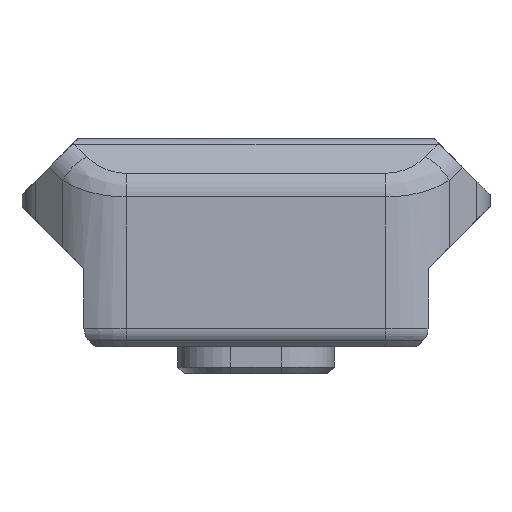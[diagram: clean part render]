
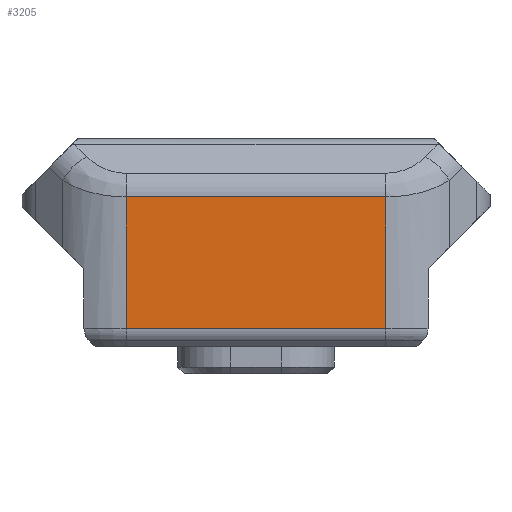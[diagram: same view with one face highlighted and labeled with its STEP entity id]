
A CAD part, front view. The second image highlights one B-rep face of the part: STEP entity #3205.
In plain terms, the highlighted planar face has unit normal (0, -1, 0).
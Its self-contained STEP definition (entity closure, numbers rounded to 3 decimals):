
#123=PLANE('',#3541);
#402=FACE_OUTER_BOUND('',#596,.T.);
#596=EDGE_LOOP('',(#2841,#2842,#2843,#2844));
#924=LINE('',#5452,#1220);
#965=LINE('',#5593,#1261);
#966=LINE('',#5597,#1262);
#967=LINE('',#5598,#1263);
#1220=VECTOR('',#4314,10.);
#1261=VECTOR('',#4437,10.);
#1262=VECTOR('',#4442,10.);
#1263=VECTOR('',#4443,10.);
#1517=VERTEX_POINT('',#5426);
#1520=VERTEX_POINT('',#5451);
#1555=VERTEX_POINT('',#5592);
#1556=VERTEX_POINT('',#5596);
#1937=EDGE_CURVE('',#1517,#1520,#924,.T.);
#1997=EDGE_CURVE('',#1517,#1555,#965,.T.);
#1999=EDGE_CURVE('',#1520,#1556,#966,.T.);
#2000=EDGE_CURVE('',#1556,#1555,#967,.T.);
#2841=ORIENTED_EDGE('',*,*,#1999,.T.);
#2842=ORIENTED_EDGE('',*,*,#2000,.T.);
#2843=ORIENTED_EDGE('',*,*,#1997,.F.);
#2844=ORIENTED_EDGE('',*,*,#1937,.T.);
#3205=ADVANCED_FACE('',(#402),#123,.T.);
#3541=AXIS2_PLACEMENT_3D('',#5595,#4440,#4441);
#4314=DIRECTION('',(0.,0.,1.));
#4437=DIRECTION('',(-1.,0.,0.));
#4440=DIRECTION('center_axis',(0.,-1.,0.));
#4441=DIRECTION('ref_axis',(1.,0.,0.));
#4442=DIRECTION('',(-1.,0.,0.));
#4443=DIRECTION('',(0.,0.,-1.));
#5426=CARTESIAN_POINT('',(5.798,-27.375,2.031));
#5451=CARTESIAN_POINT('',(5.798,-27.375,7.9));
#5452=CARTESIAN_POINT('',(5.798,-27.375,7.642));
#5592=CARTESIAN_POINT('',(-5.798,-27.375,2.031));
#5593=CARTESIAN_POINT('',(-9.762,-27.375,2.031));
#5595=CARTESIAN_POINT('Origin',(-10.455,-27.375,7.525));
#5596=CARTESIAN_POINT('',(-5.798,-27.375,7.9));
#5597=CARTESIAN_POINT('',(-9.823,-27.375,7.9));
#5598=CARTESIAN_POINT('',(-5.798,-27.375,7.642));
